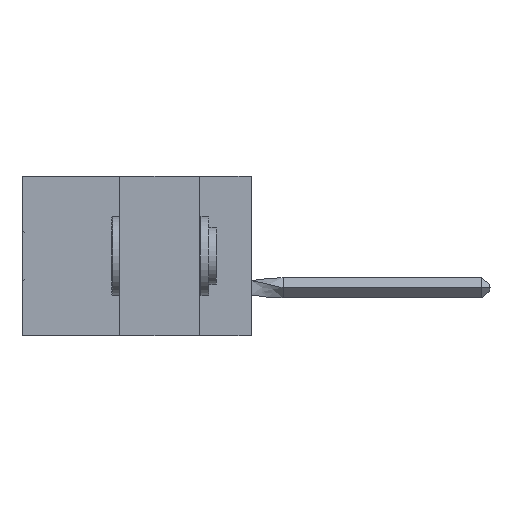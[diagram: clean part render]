
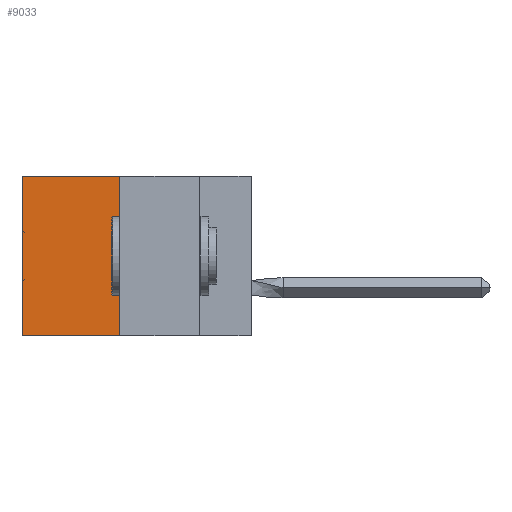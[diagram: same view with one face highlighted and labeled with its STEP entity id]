
A CAD part, left-side view. The second image highlights one B-rep face of the part: STEP entity #9033.
In plain terms, the highlighted planar face has unit normal (-1, 0, 0).
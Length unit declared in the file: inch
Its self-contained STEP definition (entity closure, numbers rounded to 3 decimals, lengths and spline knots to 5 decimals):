
#1382 = DIRECTION ( 'NONE',  ( 1., 0., 0. ) ) ;
#1616 = VERTEX_POINT ( 'NONE', #23026 ) ;
#2107 = VERTEX_POINT ( 'NONE', #36004 ) ;
#2150 = CARTESIAN_POINT ( 'NONE',  ( 0.305, 0.72, -0.5 ) ) ;
#2982 = DIRECTION ( 'NONE',  ( 0., 1., 0. ) ) ;
#5369 = DIRECTION ( 'NONE',  ( 0., 0., -1. ) ) ;
#7361 = EDGE_CURVE ( 'NONE', #2107, #1616, #29251, .T. ) ;
#9033 = ADVANCED_FACE ( 'NONE', ( #29792 ), #47139, .F. ) ;
#14216 = ORIENTED_EDGE ( 'NONE', *, *, #18847, .F. ) ;
#14310 = VECTOR ( 'NONE', #33535, 39.37008 ) ;
#14661 = LINE ( 'NONE', #52649, #19869 ) ;
#15028 = EDGE_CURVE ( 'NONE', #2107, #44340, #14661, .T. ) ;
#16704 = CARTESIAN_POINT ( 'NONE',  ( 0.305, 0.72, -0.5 ) ) ;
#18759 = EDGE_CURVE ( 'NONE', #44340, #42944, #35120, .T. ) ;
#18847 = EDGE_CURVE ( 'NONE', #1616, #42944, #22165, .T. ) ;
#19869 = VECTOR ( 'NONE', #2982, 39.37008 ) ;
#20107 = VECTOR ( 'NONE', #46840, 39.37008 ) ;
#21521 = CARTESIAN_POINT ( 'NONE',  ( 0.305, 0.413, -0.5 ) ) ;
#22165 = LINE ( 'NONE', #24607, #14310 ) ;
#23026 = CARTESIAN_POINT ( 'NONE',  ( 0.305, 0.413, -0.5 ) ) ;
#24607 = CARTESIAN_POINT ( 'NONE',  ( 0.305, 0.413, -0.5 ) ) ;
#25565 = CARTESIAN_POINT ( 'NONE',  ( 0.305, 0.413, -0.5 ) ) ;
#28219 = AXIS2_PLACEMENT_3D ( 'NONE', #21521, #1382, #5369 ) ;
#29251 = LINE ( 'NONE', #25565, #20107 ) ;
#29470 = ORIENTED_EDGE ( 'NONE', *, *, #7361, .F. ) ;
#29644 = CARTESIAN_POINT ( 'NONE',  ( 0.305, 0.72, 0. ) ) ;
#29792 = FACE_OUTER_BOUND ( 'NONE', #47670, .T. ) ;
#33188 = ORIENTED_EDGE ( 'NONE', *, *, #15028, .T. ) ;
#33535 = DIRECTION ( 'NONE',  ( 0., 1., 0. ) ) ;
#35120 = LINE ( 'NONE', #2150, #42975 ) ;
#36004 = CARTESIAN_POINT ( 'NONE',  ( 0.305, 0.413, 0. ) ) ;
#42944 = VERTEX_POINT ( 'NONE', #16704 ) ;
#42975 = VECTOR ( 'NONE', #43760, 39.37008 ) ;
#43760 = DIRECTION ( 'NONE',  ( 0., 0., -1. ) ) ;
#44340 = VERTEX_POINT ( 'NONE', #29644 ) ;
#46840 = DIRECTION ( 'NONE',  ( 0., 0., -1. ) ) ;
#47139 = PLANE ( 'NONE',  #28219 ) ;
#47670 = EDGE_LOOP ( 'NONE', ( #49723, #14216, #29470, #33188 ) ) ;
#49723 = ORIENTED_EDGE ( 'NONE', *, *, #18759, .T. ) ;
#52649 = CARTESIAN_POINT ( 'NONE',  ( 0.305, 0.413, 0. ) ) ;
